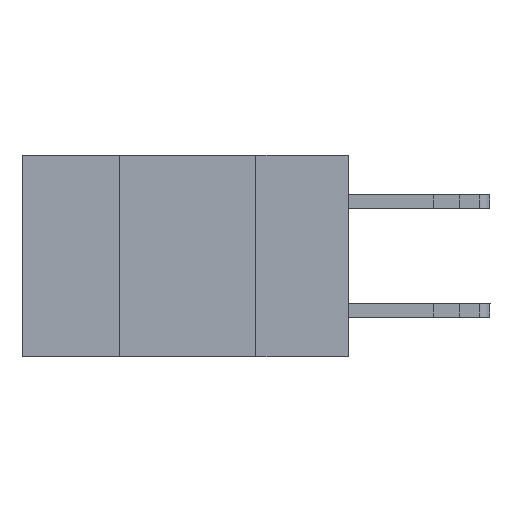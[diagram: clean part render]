
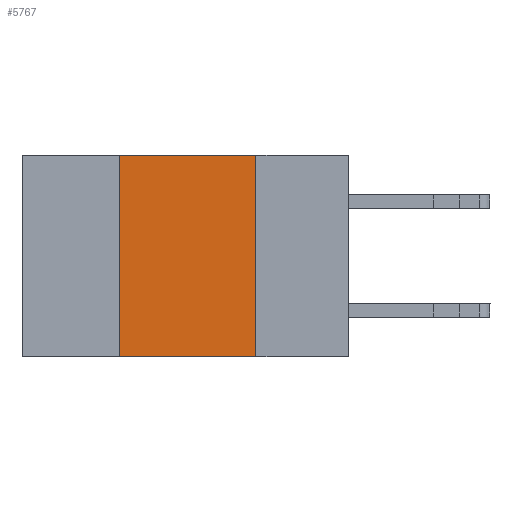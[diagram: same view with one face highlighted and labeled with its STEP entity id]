
A CAD part, left-side view. The second image highlights one B-rep face of the part: STEP entity #5767.
In plain terms, the highlighted planar face has unit normal (-1, 0, 0).
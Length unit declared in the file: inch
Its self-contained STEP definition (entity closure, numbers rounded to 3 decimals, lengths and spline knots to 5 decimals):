
#35 = LINE ( 'NONE', #2240, #5964 ) ;
#582 = CARTESIAN_POINT ( 'NONE',  ( 0., 0.42, 0. ) ) ;
#1583 = EDGE_LOOP ( 'NONE', ( #11418, #12024, #13434, #13284 ) ) ;
#1779 = EDGE_CURVE ( 'NONE', #12399, #14676, #10607, .T. ) ;
#2240 = CARTESIAN_POINT ( 'NONE',  ( 0., 0.6, 0. ) ) ;
#2702 = EDGE_CURVE ( 'NONE', #10639, #14676, #11270, .T. ) ;
#2750 = CARTESIAN_POINT ( 'NONE',  ( 0., 0.6, -0.37 ) ) ;
#3478 = CARTESIAN_POINT ( 'NONE',  ( 0., 0.17, 0. ) ) ;
#3777 = VECTOR ( 'NONE', #4970, 39.37008 ) ;
#3962 = VERTEX_POINT ( 'NONE', #582 ) ;
#4782 = AXIS2_PLACEMENT_3D ( 'NONE', #10709, #10625, #10622 ) ;
#4970 = DIRECTION ( 'NONE',  ( 0., 0., -1. ) ) ;
#5767 = ADVANCED_FACE ( 'NONE', ( #16273 ), #10728, .F. ) ;
#5964 = VECTOR ( 'NONE', #15126, 39.37008 ) ;
#6894 = CARTESIAN_POINT ( 'NONE',  ( 0., 0.42, -0.37 ) ) ;
#7213 = CARTESIAN_POINT ( 'NONE',  ( 0., 0.17, -0.37 ) ) ;
#7907 = EDGE_CURVE ( 'NONE', #10639, #3962, #10881, .T. ) ;
#8734 = DIRECTION ( 'NONE',  ( 0., -1., 0. ) ) ;
#10607 = LINE ( 'NONE', #7213, #3777 ) ;
#10622 = DIRECTION ( 'NONE',  ( 0., 0., -1. ) ) ;
#10625 = DIRECTION ( 'NONE',  ( 1., 0., 0. ) ) ;
#10639 = VERTEX_POINT ( 'NONE', #6894 ) ;
#10709 = CARTESIAN_POINT ( 'NONE',  ( 0., 0.6, 0. ) ) ;
#10728 = PLANE ( 'NONE',  #4782 ) ;
#10881 = LINE ( 'NONE', #15286, #13915 ) ;
#11270 = LINE ( 'NONE', #2750, #14261 ) ;
#11418 = ORIENTED_EDGE ( 'NONE', *, *, #1779, .F. ) ;
#12024 = ORIENTED_EDGE ( 'NONE', *, *, #15131, .F. ) ;
#12399 = VERTEX_POINT ( 'NONE', #3478 ) ;
#13284 = ORIENTED_EDGE ( 'NONE', *, *, #2702, .T. ) ;
#13434 = ORIENTED_EDGE ( 'NONE', *, *, #7907, .F. ) ;
#13915 = VECTOR ( 'NONE', #14624, 39.37008 ) ;
#14261 = VECTOR ( 'NONE', #8734, 39.37008 ) ;
#14624 = DIRECTION ( 'NONE',  ( 0., 0., 1. ) ) ;
#14676 = VERTEX_POINT ( 'NONE', #16735 ) ;
#15126 = DIRECTION ( 'NONE',  ( 0., -1., 0. ) ) ;
#15131 = EDGE_CURVE ( 'NONE', #3962, #12399, #35, .T. ) ;
#15286 = CARTESIAN_POINT ( 'NONE',  ( 0., 0.42, -0.37 ) ) ;
#16273 = FACE_OUTER_BOUND ( 'NONE', #1583, .T. ) ;
#16735 = CARTESIAN_POINT ( 'NONE',  ( 0., 0.17, -0.37 ) ) ;
